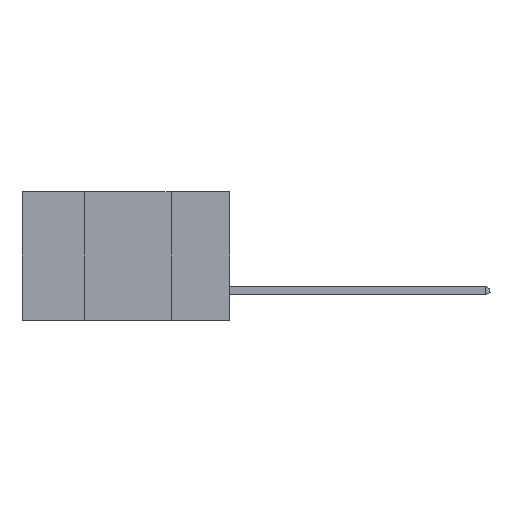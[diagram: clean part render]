
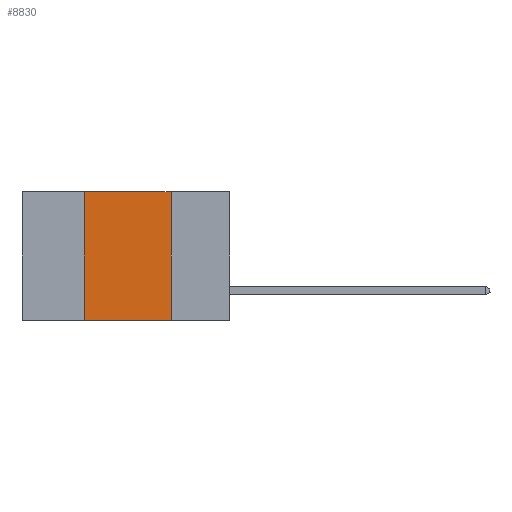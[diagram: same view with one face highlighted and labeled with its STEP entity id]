
A CAD part, left-side view. The second image highlights one B-rep face of the part: STEP entity #8830.
In plain terms, the highlighted planar face has unit normal (-1, 0, 0).
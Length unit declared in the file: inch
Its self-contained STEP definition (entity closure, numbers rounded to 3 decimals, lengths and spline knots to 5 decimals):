
#471 = CARTESIAN_POINT ( 'NONE',  ( 0., 0.17, 0. ) ) ;
#547 = VECTOR ( 'NONE', #27045, 39.37008 ) ;
#3633 = CARTESIAN_POINT ( 'NONE',  ( 0., 0.42, 0. ) ) ;
#3636 = DIRECTION ( 'NONE',  ( 0., -1., 0. ) ) ;
#4008 = CARTESIAN_POINT ( 'NONE',  ( 0., 0.6, 0. ) ) ;
#4248 = VERTEX_POINT ( 'NONE', #25022 ) ;
#4734 = ORIENTED_EDGE ( 'NONE', *, *, #10890, .F. ) ;
#5807 = AXIS2_PLACEMENT_3D ( 'NONE', #4008, #14628, #23305 ) ;
#6225 = VECTOR ( 'NONE', #8105, 39.37008 ) ;
#8105 = DIRECTION ( 'NONE',  ( 0., 0., -1. ) ) ;
#8259 = VERTEX_POINT ( 'NONE', #471 ) ;
#8830 = ADVANCED_FACE ( 'NONE', ( #12098 ), #25360, .F. ) ;
#9664 = LINE ( 'NONE', #20519, #20352 ) ;
#10143 = EDGE_CURVE ( 'NONE', #4248, #19253, #9664, .T. ) ;
#10890 = EDGE_CURVE ( 'NONE', #4248, #26688, #12303, .T. ) ;
#11340 = EDGE_CURVE ( 'NONE', #8259, #19253, #24633, .T. ) ;
#11450 = CARTESIAN_POINT ( 'NONE',  ( 0., 0.42, 0. ) ) ;
#12098 = FACE_OUTER_BOUND ( 'NONE', #24825, .T. ) ;
#12263 = LINE ( 'NONE', #22559, #18960 ) ;
#12303 = LINE ( 'NONE', #3633, #547 ) ;
#14628 = DIRECTION ( 'NONE',  ( 1., 0., 0. ) ) ;
#17439 = EDGE_CURVE ( 'NONE', #26688, #8259, #12263, .T. ) ;
#18960 = VECTOR ( 'NONE', #22660, 39.37008 ) ;
#19165 = ORIENTED_EDGE ( 'NONE', *, *, #10143, .T. ) ;
#19253 = VERTEX_POINT ( 'NONE', #22616 ) ;
#20352 = VECTOR ( 'NONE', #3636, 39.37008 ) ;
#20519 = CARTESIAN_POINT ( 'NONE',  ( 0., 0.6, -0.37 ) ) ;
#22559 = CARTESIAN_POINT ( 'NONE',  ( 0., 0.6, 0. ) ) ;
#22616 = CARTESIAN_POINT ( 'NONE',  ( 0., 0.17, -0.37 ) ) ;
#22660 = DIRECTION ( 'NONE',  ( 0., -1., 0. ) ) ;
#22780 = CARTESIAN_POINT ( 'NONE',  ( 0., 0.17, 0. ) ) ;
#23305 = DIRECTION ( 'NONE',  ( 0., 0., -1. ) ) ;
#24633 = LINE ( 'NONE', #22780, #6225 ) ;
#24777 = ORIENTED_EDGE ( 'NONE', *, *, #11340, .F. ) ;
#24825 = EDGE_LOOP ( 'NONE', ( #24777, #27503, #4734, #19165 ) ) ;
#25022 = CARTESIAN_POINT ( 'NONE',  ( 0., 0.42, -0.37 ) ) ;
#25360 = PLANE ( 'NONE',  #5807 ) ;
#26688 = VERTEX_POINT ( 'NONE', #11450 ) ;
#27045 = DIRECTION ( 'NONE',  ( 0., 0., 1. ) ) ;
#27503 = ORIENTED_EDGE ( 'NONE', *, *, #17439, .F. ) ;
